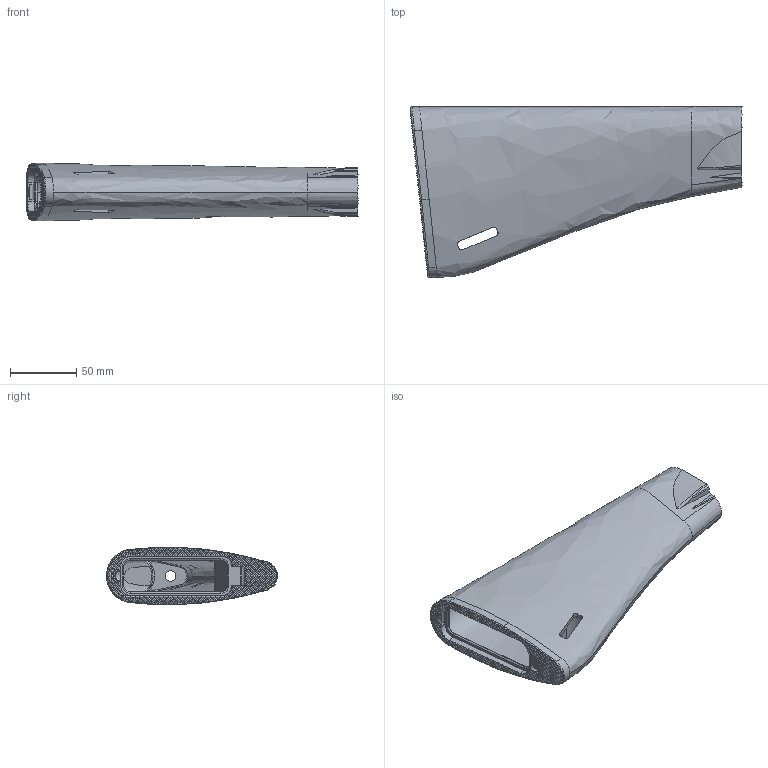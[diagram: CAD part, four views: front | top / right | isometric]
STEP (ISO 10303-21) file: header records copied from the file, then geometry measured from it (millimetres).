
FILE_DESCRIPTION (( 'STEP AP203' ), '1' );
FILE_NAME ('mbbi_monolithic_rear.STEP', '2022-06-11T19:58:07', ( '' ), ( '' ), 'SwSTEP 2.0', 'SolidWorks 2021', '' );
FILE_SCHEMA (( 'CONFIG_CONTROL_DESIGN' ));
Products named in the file (1): mbbi_monolithic_rear
Bounding box: 251.48 x 129.54 x 43.56 mm (x, y, z)
Volume: 245754.5 mm3; surface area: 124824.2 mm2
Topology: 1 solids, 1 shells, 1889 faces, 5210 edges, 3436 vertices
Faces by surface type: plane 1753, cylinder 64, bspline 49, torus 14, sphere 9
Entity records: 71719 total; most frequent: CARTESIAN_POINT 31117, ORIENTED_EDGE 10404, DIRECTION 5312, EDGE_CURVE 5202, B_SPLINE_CURVE_WITH_KNOTS 3586, VERTEX_POINT 3432, EDGE_LOOP 2012, AXIS2_PLACEMENT_3D 1988
